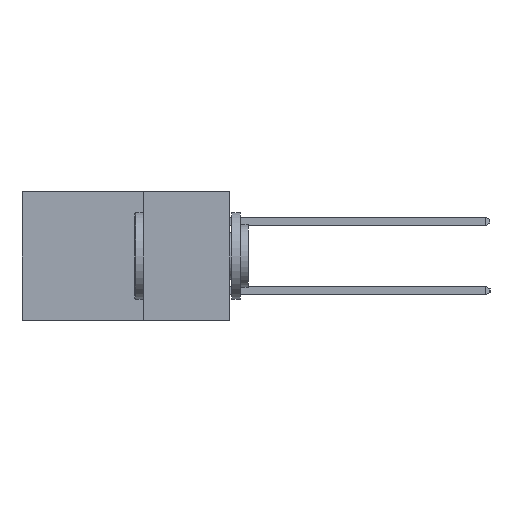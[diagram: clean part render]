
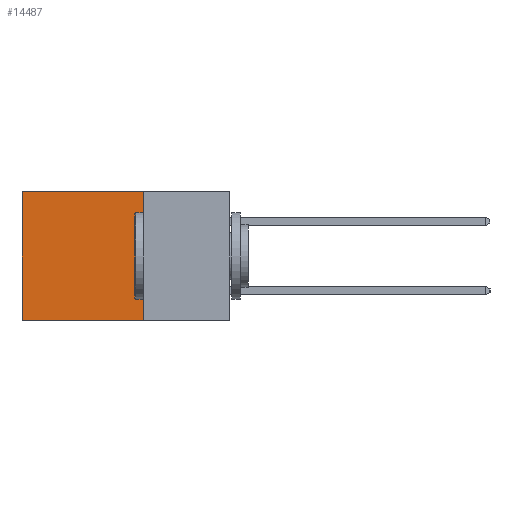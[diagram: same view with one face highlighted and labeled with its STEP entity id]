
A CAD part, left-side view. The second image highlights one B-rep face of the part: STEP entity #14487.
In plain terms, the highlighted planar face has unit normal (-1, 0, 0).
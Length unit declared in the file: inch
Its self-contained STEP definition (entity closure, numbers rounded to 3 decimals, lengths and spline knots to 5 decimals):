
#95 = LINE ( 'NONE', #22938, #20394 ) ;
#138 = LINE ( 'NONE', #20962, #15376 ) ;
#1359 = VECTOR ( 'NONE', #6950, 39.37008 ) ;
#2523 = DIRECTION ( 'NONE',  ( 1., 0., 0. ) ) ;
#3144 = ORIENTED_EDGE ( 'NONE', *, *, #23868, .T. ) ;
#3314 = CARTESIAN_POINT ( 'NONE',  ( 0.2615, 0.25, -0.37 ) ) ;
#4674 = CARTESIAN_POINT ( 'NONE',  ( 0.2615, 0.25, 0. ) ) ;
#5483 = DIRECTION ( 'NONE',  ( 0., 1., 0. ) ) ;
#6006 = VERTEX_POINT ( 'NONE', #6531 ) ;
#6117 = VERTEX_POINT ( 'NONE', #3314 ) ;
#6216 = FACE_OUTER_BOUND ( 'NONE', #16937, .T. ) ;
#6531 = CARTESIAN_POINT ( 'NONE',  ( 0.2615, 0.6, -0.37 ) ) ;
#6950 = DIRECTION ( 'NONE',  ( 0., 1., 0. ) ) ;
#6956 = AXIS2_PLACEMENT_3D ( 'NONE', #12428, #2523, #16394 ) ;
#7588 = EDGE_CURVE ( 'NONE', #13865, #6117, #138, .T. ) ;
#10417 = ORIENTED_EDGE ( 'NONE', *, *, #18581, .T. ) ;
#11928 = LINE ( 'NONE', #16810, #1359 ) ;
#12428 = CARTESIAN_POINT ( 'NONE',  ( 0.2615, 0.25, -0.37 ) ) ;
#13865 = VERTEX_POINT ( 'NONE', #4674 ) ;
#14406 = PLANE ( 'NONE',  #6956 ) ;
#14487 = ADVANCED_FACE ( 'NONE', ( #6216 ), #14406, .F. ) ;
#15100 = LINE ( 'NONE', #17983, #24525 ) ;
#15376 = VECTOR ( 'NONE', #22835, 39.37008 ) ;
#16101 = VERTEX_POINT ( 'NONE', #19509 ) ;
#16394 = DIRECTION ( 'NONE',  ( 0., 0., -1. ) ) ;
#16810 = CARTESIAN_POINT ( 'NONE',  ( 0.2615, 0.25, -0.37 ) ) ;
#16937 = EDGE_LOOP ( 'NONE', ( #3144, #23996, #22235, #10417 ) ) ;
#17983 = CARTESIAN_POINT ( 'NONE',  ( 0.2615, 0.6, -0.37 ) ) ;
#18063 = DIRECTION ( 'NONE',  ( 0., 0., -1. ) ) ;
#18581 = EDGE_CURVE ( 'NONE', #13865, #16101, #95, .T. ) ;
#18765 = EDGE_CURVE ( 'NONE', #6117, #6006, #11928, .T. ) ;
#19509 = CARTESIAN_POINT ( 'NONE',  ( 0.2615, 0.6, 0. ) ) ;
#20394 = VECTOR ( 'NONE', #5483, 39.37008 ) ;
#20962 = CARTESIAN_POINT ( 'NONE',  ( 0.2615, 0.25, -0.37 ) ) ;
#22235 = ORIENTED_EDGE ( 'NONE', *, *, #7588, .F. ) ;
#22835 = DIRECTION ( 'NONE',  ( 0., 0., -1. ) ) ;
#22938 = CARTESIAN_POINT ( 'NONE',  ( 0.2615, 0.25, 0. ) ) ;
#23868 = EDGE_CURVE ( 'NONE', #16101, #6006, #15100, .T. ) ;
#23996 = ORIENTED_EDGE ( 'NONE', *, *, #18765, .F. ) ;
#24525 = VECTOR ( 'NONE', #18063, 39.37008 ) ;
